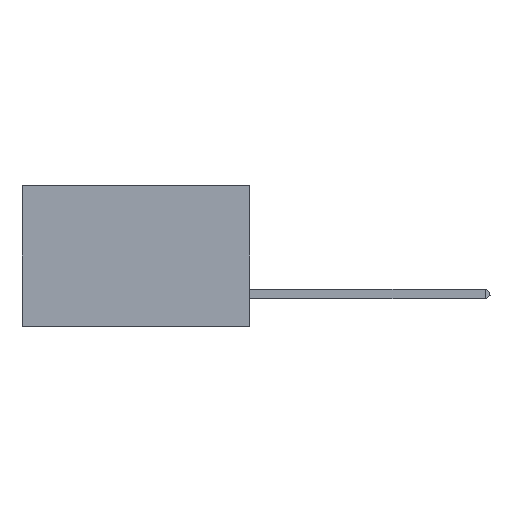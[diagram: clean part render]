
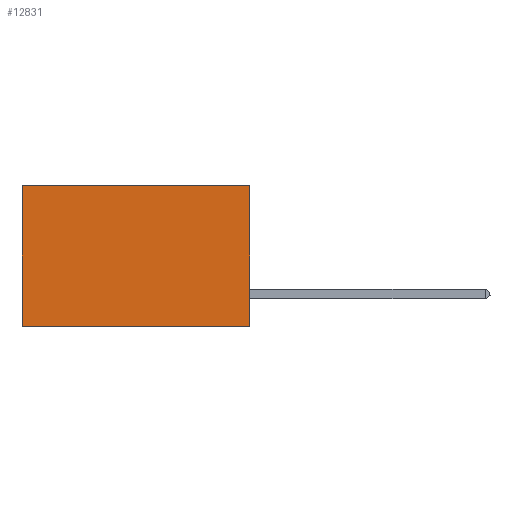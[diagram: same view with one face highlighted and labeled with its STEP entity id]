
A CAD part, left-side view. The second image highlights one B-rep face of the part: STEP entity #12831.
In plain terms, the highlighted planar face has unit normal (-1, 0, 0).
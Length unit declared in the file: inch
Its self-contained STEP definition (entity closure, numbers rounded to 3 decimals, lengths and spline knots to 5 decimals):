
#760 = VECTOR ( 'NONE', #4837, 39.37008 ) ;
#797 = CARTESIAN_POINT ( 'NONE',  ( 0.2875, 0., 0. ) ) ;
#1205 = ORIENTED_EDGE ( 'NONE', *, *, #5339, .F. ) ;
#1698 = CARTESIAN_POINT ( 'NONE',  ( 0.2875, 0., -0.37 ) ) ;
#2041 = AXIS2_PLACEMENT_3D ( 'NONE', #10154, #3988, #11208 ) ;
#2887 = LINE ( 'NONE', #12995, #7886 ) ;
#3126 = EDGE_CURVE ( 'NONE', #7760, #7707, #2887, .T. ) ;
#3811 = VECTOR ( 'NONE', #5646, 39.37008 ) ;
#3827 = EDGE_CURVE ( 'NONE', #10942, #10552, #12745, .T. ) ;
#3988 = DIRECTION ( 'NONE',  ( 1., 0., 0. ) ) ;
#4188 = ORIENTED_EDGE ( 'NONE', *, *, #13167, .T. ) ;
#4647 = DIRECTION ( 'NONE',  ( 0., 0., -1. ) ) ;
#4837 = DIRECTION ( 'NONE',  ( 0., 0., -1. ) ) ;
#4941 = CARTESIAN_POINT ( 'NONE',  ( 0.2875, 0., 0. ) ) ;
#5326 = CARTESIAN_POINT ( 'NONE',  ( 0.2875, 0.6, 0. ) ) ;
#5339 = EDGE_CURVE ( 'NONE', #10552, #7707, #12698, .T. ) ;
#5646 = DIRECTION ( 'NONE',  ( 0., 1., 0. ) ) ;
#6799 = ORIENTED_EDGE ( 'NONE', *, *, #3827, .F. ) ;
#6966 = DIRECTION ( 'NONE',  ( 0., 1., 0. ) ) ;
#7081 = ORIENTED_EDGE ( 'NONE', *, *, #3126, .T. ) ;
#7145 = CARTESIAN_POINT ( 'NONE',  ( 0.2875, 0., -0.37 ) ) ;
#7707 = VERTEX_POINT ( 'NONE', #9406 ) ;
#7760 = VERTEX_POINT ( 'NONE', #5326 ) ;
#7886 = VECTOR ( 'NONE', #4647, 39.37008 ) ;
#9406 = CARTESIAN_POINT ( 'NONE',  ( 0.2875, 0.6, -0.37 ) ) ;
#9575 = FACE_OUTER_BOUND ( 'NONE', #9937, .T. ) ;
#9937 = EDGE_LOOP ( 'NONE', ( #7081, #1205, #6799, #4188 ) ) ;
#10154 = CARTESIAN_POINT ( 'NONE',  ( 0.2875, 0., 0. ) ) ;
#10193 = LINE ( 'NONE', #11308, #12631 ) ;
#10552 = VERTEX_POINT ( 'NONE', #7145 ) ;
#10942 = VERTEX_POINT ( 'NONE', #4941 ) ;
#11208 = DIRECTION ( 'NONE',  ( 0., 0., -1. ) ) ;
#11308 = CARTESIAN_POINT ( 'NONE',  ( 0.2875, 0., 0. ) ) ;
#12021 = PLANE ( 'NONE',  #2041 ) ;
#12631 = VECTOR ( 'NONE', #6966, 39.37008 ) ;
#12698 = LINE ( 'NONE', #1698, #3811 ) ;
#12745 = LINE ( 'NONE', #797, #760 ) ;
#12831 = ADVANCED_FACE ( 'NONE', ( #9575 ), #12021, .F. ) ;
#12995 = CARTESIAN_POINT ( 'NONE',  ( 0.2875, 0.6, 0. ) ) ;
#13167 = EDGE_CURVE ( 'NONE', #10942, #7760, #10193, .T. ) ;
